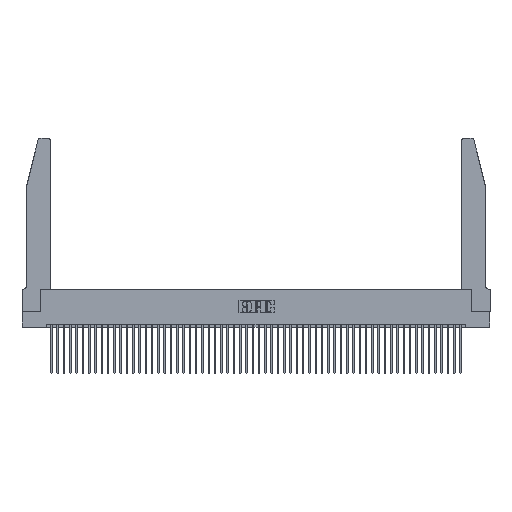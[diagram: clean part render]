
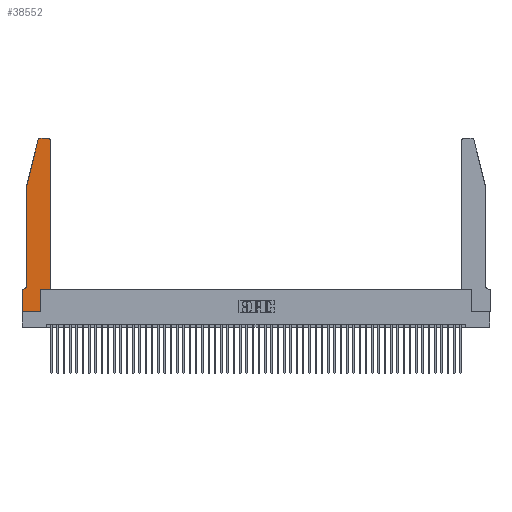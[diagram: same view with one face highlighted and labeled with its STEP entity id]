
A CAD part, top view. The second image highlights one B-rep face of the part: STEP entity #38552.
In plain terms, the highlighted planar face has unit normal (0, 0, 1).
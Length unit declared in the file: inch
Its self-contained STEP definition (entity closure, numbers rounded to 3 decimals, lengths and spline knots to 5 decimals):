
#265 = LINE ( 'NONE', #9284, #2218 ) ;
#979 = CIRCLE ( 'NONE', #21129, 0.07 ) ;
#1354 = DIRECTION ( 'NONE',  ( 0., 1., 0. ) ) ;
#1865 = CARTESIAN_POINT ( 'NONE',  ( 0., 0.35, 0.37 ) ) ;
#2218 = VECTOR ( 'NONE', #5304, 39.37008 ) ;
#2895 = DIRECTION ( 'NONE',  ( 0., 0., 1. ) ) ;
#4386 = ORIENTED_EDGE ( 'NONE', *, *, #30459, .T. ) ;
#4550 = CARTESIAN_POINT ( 'NONE',  ( 0., 0., 0.37 ) ) ;
#4614 = LINE ( 'NONE', #40534, #44548 ) ;
#4883 = CARTESIAN_POINT ( 'NONE',  ( 0.4205, 2.75, 0.37 ) ) ;
#5288 = VECTOR ( 'NONE', #12051, 39.37008 ) ;
#5304 = DIRECTION ( 'NONE',  ( 0., 1., 0. ) ) ;
#5361 = VERTEX_POINT ( 'NONE', #49579 ) ;
#5531 = VERTEX_POINT ( 'NONE', #1865 ) ;
#6191 = ORIENTED_EDGE ( 'NONE', *, *, #48993, .T. ) ;
#7120 = EDGE_CURVE ( 'NONE', #17974, #33210, #265, .T. ) ;
#7460 = DIRECTION ( 'NONE',  ( 1., 0., 0. ) ) ;
#7945 = VERTEX_POINT ( 'NONE', #4883 ) ;
#8838 = DIRECTION ( 'NONE',  ( 1., 0., 0. ) ) ;
#9134 = AXIS2_PLACEMENT_3D ( 'NONE', #37423, #17284, #8838 ) ;
#9284 = CARTESIAN_POINT ( 'NONE',  ( 0.2865, 0.35, 0.37 ) ) ;
#10116 = VERTEX_POINT ( 'NONE', #22880 ) ;
#10393 = CARTESIAN_POINT ( 'NONE',  ( 0.0055, 0.42, 0.37 ) ) ;
#10469 = DIRECTION ( 'NONE',  ( 0., -1., 0. ) ) ;
#11773 = FACE_OUTER_BOUND ( 'NONE', #25091, .T. ) ;
#11926 = CARTESIAN_POINT ( 'NONE',  ( 0.284, 2.75, 0.37 ) ) ;
#12051 = DIRECTION ( 'NONE',  ( -1., 0., 0. ) ) ;
#12895 = ORIENTED_EDGE ( 'NONE', *, *, #45182, .T. ) ;
#14289 = CARTESIAN_POINT ( 'NONE',  ( 0.0755, 2., 0.37 ) ) ;
#14554 = VERTEX_POINT ( 'NONE', #11926 ) ;
#14995 = VERTEX_POINT ( 'NONE', #51331 ) ;
#15391 = VECTOR ( 'NONE', #43047, 39.37008 ) ;
#15417 = DIRECTION ( 'NONE',  ( 0., -1., 0. ) ) ;
#16023 = CARTESIAN_POINT ( 'NONE',  ( 0.0755, 0.35, 0.37 ) ) ;
#17284 = DIRECTION ( 'NONE',  ( 0., 0., 1. ) ) ;
#17647 = LINE ( 'NONE', #39399, #20220 ) ;
#17974 = VERTEX_POINT ( 'NONE', #40093 ) ;
#18301 = CARTESIAN_POINT ( 'NONE',  ( 0.284, 2.72, 0.37 ) ) ;
#18976 = CARTESIAN_POINT ( 'NONE',  ( 0.4205, 2.72, 0.37 ) ) ;
#18980 = EDGE_CURVE ( 'NONE', #33210, #20708, #4614, .T. ) ;
#19503 = VECTOR ( 'NONE', #29188, 39.37008 ) ;
#20220 = VECTOR ( 'NONE', #10469, 39.37008 ) ;
#20708 = VERTEX_POINT ( 'NONE', #26570 ) ;
#21129 = AXIS2_PLACEMENT_3D ( 'NONE', #10393, #51928, #43296 ) ;
#22495 = LINE ( 'NONE', #14289, #15391 ) ;
#22880 = CARTESIAN_POINT ( 'NONE',  ( 0.0755, 2., 0.37 ) ) ;
#22928 = ORIENTED_EDGE ( 'NONE', *, *, #27825, .T. ) ;
#23425 = EDGE_CURVE ( 'NONE', #14995, #17974, #27816, .T. ) ;
#24876 = CARTESIAN_POINT ( 'NONE',  ( 0.2865, 0.35, 0.37 ) ) ;
#25091 = EDGE_LOOP ( 'NONE', ( #6191, #22928, #12895, #26605, #46917, #43663, #42488, #25802, #51656, #41524, #4386, #37397 ) ) ;
#25802 = ORIENTED_EDGE ( 'NONE', *, *, #23425, .T. ) ;
#26018 = DIRECTION ( 'NONE',  ( 1., 0., 0. ) ) ;
#26329 = CIRCLE ( 'NONE', #36666, 0.03 ) ;
#26570 = CARTESIAN_POINT ( 'NONE',  ( 0.4505, 0.35, 0.37 ) ) ;
#26605 = ORIENTED_EDGE ( 'NONE', *, *, #41548, .T. ) ;
#26696 = LINE ( 'NONE', #37910, #41478 ) ;
#27816 = LINE ( 'NONE', #4550, #19503 ) ;
#27825 = EDGE_CURVE ( 'NONE', #14554, #44488, #26329, .T. ) ;
#29188 = DIRECTION ( 'NONE',  ( 1., 0., 0. ) ) ;
#29707 = EDGE_CURVE ( 'NONE', #49908, #5531, #30619, .T. ) ;
#30459 = EDGE_CURVE ( 'NONE', #20708, #5361, #26696, .T. ) ;
#30619 = LINE ( 'NONE', #16023, #33179 ) ;
#31753 = LINE ( 'NONE', #40388, #53030 ) ;
#31843 = CARTESIAN_POINT ( 'NONE',  ( 0.0755, 0.42, 0.37 ) ) ;
#32016 = CARTESIAN_POINT ( 'NONE',  ( 0.2605, 2.75, 0.37 ) ) ;
#33121 = AXIS2_PLACEMENT_3D ( 'NONE', #18976, #2895, #48395 ) ;
#33179 = VECTOR ( 'NONE', #40472, 39.37008 ) ;
#33210 = VERTEX_POINT ( 'NONE', #24876 ) ;
#33454 = PLANE ( 'NONE',  #9134 ) ;
#33848 = CARTESIAN_POINT ( 'NONE',  ( 0.0055, 0.35, 0.37 ) ) ;
#34435 = CIRCLE ( 'NONE', #33121, 0.03 ) ;
#36080 = EDGE_CURVE ( 'NONE', #45330, #49908, #979, .T. ) ;
#36666 = AXIS2_PLACEMENT_3D ( 'NONE', #18301, #47084, #26018 ) ;
#37397 = ORIENTED_EDGE ( 'NONE', *, *, #52917, .T. ) ;
#37423 = CARTESIAN_POINT ( 'NONE',  ( 0., 0.35, 0.37 ) ) ;
#37910 = CARTESIAN_POINT ( 'NONE',  ( 0.4505, 0.35, 0.37 ) ) ;
#38552 = ADVANCED_FACE ( 'NONE', ( #11773 ), #33454, .T. ) ;
#39399 = CARTESIAN_POINT ( 'NONE',  ( 0.0755, 2., 0.37 ) ) ;
#40093 = CARTESIAN_POINT ( 'NONE',  ( 0.2865, 0., 0.37 ) ) ;
#40388 = CARTESIAN_POINT ( 'NONE',  ( 0., 0., 0.37 ) ) ;
#40472 = DIRECTION ( 'NONE',  ( -1., 0., 0. ) ) ;
#40534 = CARTESIAN_POINT ( 'NONE',  ( 0.4505, 0.35, 0.37 ) ) ;
#41478 = VECTOR ( 'NONE', #1354, 39.37008 ) ;
#41524 = ORIENTED_EDGE ( 'NONE', *, *, #18980, .T. ) ;
#41548 = EDGE_CURVE ( 'NONE', #10116, #45330, #17647, .T. ) ;
#41834 = CARTESIAN_POINT ( 'NONE',  ( 0.25487, 2.72718, 0.37 ) ) ;
#42488 = ORIENTED_EDGE ( 'NONE', *, *, #47722, .T. ) ;
#43047 = DIRECTION ( 'NONE',  ( -0.239, -0.971, 0. ) ) ;
#43296 = DIRECTION ( 'NONE',  ( -1., 0., 0. ) ) ;
#43663 = ORIENTED_EDGE ( 'NONE', *, *, #29707, .T. ) ;
#44488 = VERTEX_POINT ( 'NONE', #41834 ) ;
#44548 = VECTOR ( 'NONE', #7460, 39.37008 ) ;
#45182 = EDGE_CURVE ( 'NONE', #44488, #10116, #22495, .T. ) ;
#45330 = VERTEX_POINT ( 'NONE', #31843 ) ;
#45812 = LINE ( 'NONE', #32016, #5288 ) ;
#46917 = ORIENTED_EDGE ( 'NONE', *, *, #36080, .T. ) ;
#47084 = DIRECTION ( 'NONE',  ( 0., 0., 1. ) ) ;
#47722 = EDGE_CURVE ( 'NONE', #5531, #14995, #31753, .T. ) ;
#48395 = DIRECTION ( 'NONE',  ( 1., 0., 0. ) ) ;
#48993 = EDGE_CURVE ( 'NONE', #7945, #14554, #45812, .T. ) ;
#49579 = CARTESIAN_POINT ( 'NONE',  ( 0.4505, 2.72, 0.37 ) ) ;
#49908 = VERTEX_POINT ( 'NONE', #33848 ) ;
#51331 = CARTESIAN_POINT ( 'NONE',  ( 0., 0., 0.37 ) ) ;
#51656 = ORIENTED_EDGE ( 'NONE', *, *, #7120, .T. ) ;
#51928 = DIRECTION ( 'NONE',  ( 0., 0., -1. ) ) ;
#52917 = EDGE_CURVE ( 'NONE', #5361, #7945, #34435, .T. ) ;
#53030 = VECTOR ( 'NONE', #15417, 39.37008 ) ;
